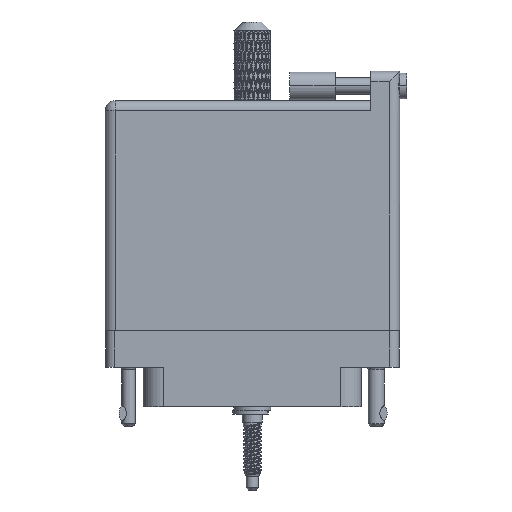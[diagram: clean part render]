
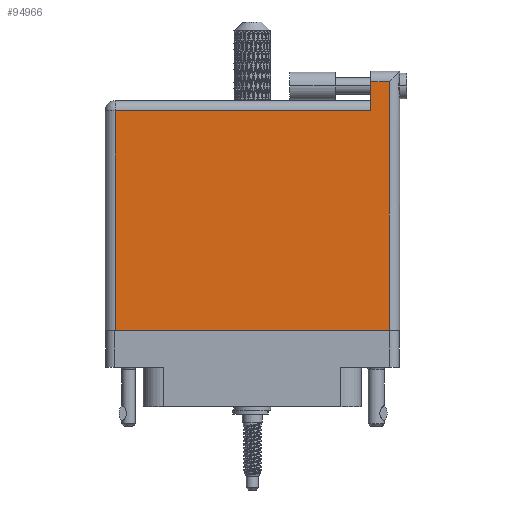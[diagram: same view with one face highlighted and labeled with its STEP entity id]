
A CAD part, front view. The second image highlights one B-rep face of the part: STEP entity #94966.
In plain terms, the highlighted face is planar.
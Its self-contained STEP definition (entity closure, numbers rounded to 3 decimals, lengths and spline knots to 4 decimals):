
#2504 = DIRECTION ( 'NONE',  ( -1., 0., 0. ) ) ;
#3623 = CARTESIAN_POINT ( 'NONE',  ( -1.004, 1.396, 0.4495 ) ) ;
#6789 = DIRECTION ( 'NONE',  ( 1., 0., 0. ) ) ;
#8383 = DIRECTION ( 'NONE',  ( 0., -1., 0. ) ) ;
#8975 = VECTOR ( 'NONE', #8383, 39.3701 ) ;
#12528 = DIRECTION ( 'NONE',  ( 0., 1., 0. ) ) ;
#13483 = VECTOR ( 'NONE', #114842, 39.3701 ) ;
#13700 = CARTESIAN_POINT ( 'NONE',  ( 0.807, 1.396, 0.4495 ) ) ;
#14592 = LINE ( 'NONE', #30285, #20687 ) ;
#19601 = VERTEX_POINT ( 'NONE', #57649 ) ;
#20687 = VECTOR ( 'NONE', #74431, 39.3701 ) ;
#22633 = ORIENTED_EDGE ( 'NONE', *, *, #63960, .T. ) ;
#23504 = CARTESIAN_POINT ( 'NONE',  ( 0.934, 1.666, 0.4495 ) ) ;
#25127 = VERTEX_POINT ( 'NONE', #99063 ) ;
#30285 = CARTESIAN_POINT ( 'NONE',  ( 0.807, 1.666, 0.4495 ) ) ;
#30838 = CARTESIAN_POINT ( 'NONE',  ( 0.807, 1.596, 0.4495 ) ) ;
#33604 = ORIENTED_EDGE ( 'NONE', *, *, #63492, .T. ) ;
#34620 = DIRECTION ( 'NONE',  ( -1., 0., 0. ) ) ;
#41905 = VERTEX_POINT ( 'NONE', #67737 ) ;
#43278 = VECTOR ( 'NONE', #6789, 39.3701 ) ;
#44514 = CARTESIAN_POINT ( 'NONE',  ( -1.004, 1.596, 0.4495 ) ) ;
#46975 = VECTOR ( 'NONE', #2504, 39.3701 ) ;
#49526 = VERTEX_POINT ( 'NONE', #13700 ) ;
#56222 = EDGE_CURVE ( 'NONE', #25127, #103896, #70095, .T. ) ;
#56940 = ORIENTED_EDGE ( 'NONE', *, *, #107070, .T. ) ;
#57649 = CARTESIAN_POINT ( 'NONE',  ( -0.934, 1.396, 0.4495 ) ) ;
#57757 = ORIENTED_EDGE ( 'NONE', *, *, #114272, .T. ) ;
#63492 = EDGE_CURVE ( 'NONE', #83532, #41905, #104360, .T. ) ;
#63960 = EDGE_CURVE ( 'NONE', #49526, #19601, #74518, .T. ) ;
#67737 = CARTESIAN_POINT ( 'NONE',  ( 0.934, -0.1, 0.4495 ) ) ;
#68877 = PLANE ( 'NONE',  #89680 ) ;
#69936 = LINE ( 'NONE', #96636, #8975 ) ;
#70095 = LINE ( 'NONE', #44514, #13483 ) ;
#74431 = DIRECTION ( 'NONE',  ( 0., -1., 0. ) ) ;
#74518 = LINE ( 'NONE', #3623, #46975 ) ;
#78758 = FACE_OUTER_BOUND ( 'NONE', #83704, .T. ) ;
#78959 = EDGE_CURVE ( 'NONE', #19601, #83532, #69936, .T. ) ;
#79406 = CARTESIAN_POINT ( 'NONE',  ( -0.934, -0.1, 0.4495 ) ) ;
#81391 = VECTOR ( 'NONE', #12528, 39.3701 ) ;
#83532 = VERTEX_POINT ( 'NONE', #79406 ) ;
#83704 = EDGE_LOOP ( 'NONE', ( #33604, #56940, #89015, #57757, #22633, #102776 ) ) ;
#86359 = CARTESIAN_POINT ( 'NONE',  ( -1.004, -0.1, 0.4495 ) ) ;
#89015 = ORIENTED_EDGE ( 'NONE', *, *, #56222, .T. ) ;
#89680 = AXIS2_PLACEMENT_3D ( 'NONE', #95025, #113629, #34620 ) ;
#93791 = LINE ( 'NONE', #23504, #81391 ) ;
#94966 = ADVANCED_FACE ( 'NONE', ( #78758 ), #68877, .F. ) ;
#95025 = CARTESIAN_POINT ( 'NONE',  ( -1.004, 1.466, 0.4495 ) ) ;
#96636 = CARTESIAN_POINT ( 'NONE',  ( -0.934, -0.1, 0.4495 ) ) ;
#99063 = CARTESIAN_POINT ( 'NONE',  ( 0.934, 1.596, 0.4495 ) ) ;
#102776 = ORIENTED_EDGE ( 'NONE', *, *, #78959, .T. ) ;
#103896 = VERTEX_POINT ( 'NONE', #30838 ) ;
#104360 = LINE ( 'NONE', #86359, #43278 ) ;
#107070 = EDGE_CURVE ( 'NONE', #41905, #25127, #93791, .T. ) ;
#113629 = DIRECTION ( 'NONE',  ( 0., 0., -1. ) ) ;
#114272 = EDGE_CURVE ( 'NONE', #103896, #49526, #14592, .T. ) ;
#114842 = DIRECTION ( 'NONE',  ( -1., 0., 0. ) ) ;
